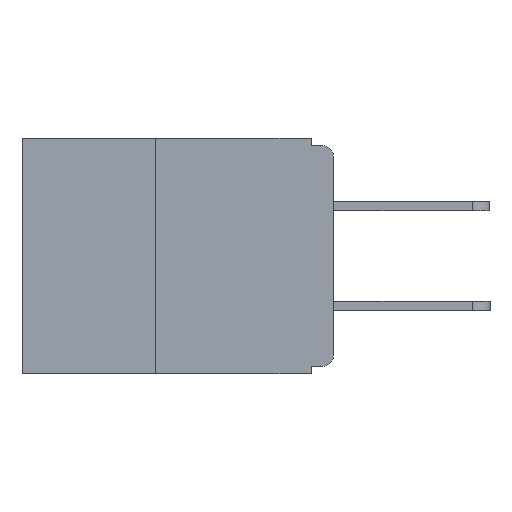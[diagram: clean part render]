
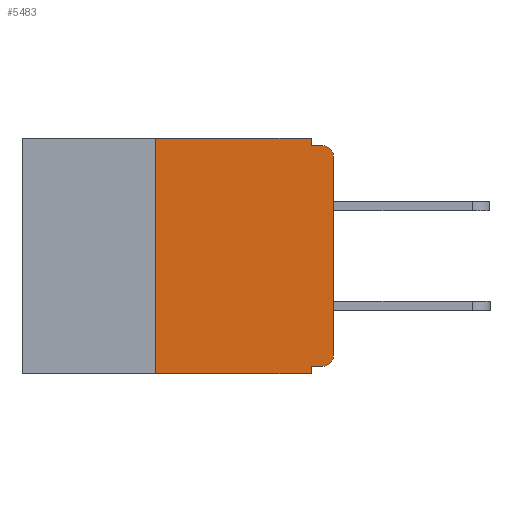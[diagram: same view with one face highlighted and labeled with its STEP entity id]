
A CAD part, left-side view. The second image highlights one B-rep face of the part: STEP entity #5483.
In plain terms, the highlighted planar face has unit normal (-1, 0, 0).
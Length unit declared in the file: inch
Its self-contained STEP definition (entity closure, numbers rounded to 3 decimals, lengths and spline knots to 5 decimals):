
#93 = EDGE_CURVE ( 'NONE', #1629, #9527, #11189, .T. ) ;
#175 = EDGE_CURVE ( 'NONE', #1629, #6311, #10903, .T. ) ;
#195 = AXIS2_PLACEMENT_3D ( 'NONE', #8005, #7891, #7655 ) ;
#348 = CARTESIAN_POINT ( 'NONE',  ( 0., 0.25, 0. ) ) ;
#1002 = CARTESIAN_POINT ( 'NONE',  ( 0., 0., -0.305 ) ) ;
#1053 = EDGE_CURVE ( 'NONE', #9122, #11343, #7869, .T. ) ;
#1329 = EDGE_CURVE ( 'NONE', #2762, #2732, #7465, .T. ) ;
#1629 = VERTEX_POINT ( 'NONE', #6068 ) ;
#1661 = AXIS2_PLACEMENT_3D ( 'NONE', #4460, #2580, #2341 ) ;
#1806 = VECTOR ( 'NONE', #8333, 39.37008 ) ;
#1836 = EDGE_CURVE ( 'NONE', #3424, #6311, #6360, .T. ) ;
#1947 = LINE ( 'NONE', #6629, #1806 ) ;
#2341 = DIRECTION ( 'NONE',  ( 0., 0., -1. ) ) ;
#2580 = DIRECTION ( 'NONE',  ( 1., 0., 0. ) ) ;
#2732 = VERTEX_POINT ( 'NONE', #11090 ) ;
#2762 = VERTEX_POINT ( 'NONE', #10242 ) ;
#2936 = DIRECTION ( 'NONE',  ( 0., 0., 1. ) ) ;
#3141 = ORIENTED_EDGE ( 'NONE', *, *, #1836, .F. ) ;
#3287 = VERTEX_POINT ( 'NONE', #11922 ) ;
#3313 = CARTESIAN_POINT ( 'NONE',  ( 0., 0.437, -0.33 ) ) ;
#3424 = VERTEX_POINT ( 'NONE', #4316 ) ;
#3521 = EDGE_CURVE ( 'NONE', #9527, #9820, #1947, .T. ) ;
#3797 = ORIENTED_EDGE ( 'NONE', *, *, #175, .T. ) ;
#4178 = EDGE_CURVE ( 'NONE', #9122, #3424, #12472, .T. ) ;
#4255 = EDGE_CURVE ( 'NONE', #11343, #3287, #12326, .T. ) ;
#4316 = CARTESIAN_POINT ( 'NONE',  ( 0., 0.031, -0.32 ) ) ;
#4460 = CARTESIAN_POINT ( 'NONE',  ( 0., 0.437, 0. ) ) ;
#4628 = PLANE ( 'NONE',  #1661 ) ;
#5052 = CARTESIAN_POINT ( 'NONE',  ( 0., 0.015, -0.32 ) ) ;
#5068 = ORIENTED_EDGE ( 'NONE', *, *, #93, .F. ) ;
#5282 = DIRECTION ( 'NONE',  ( 0., -1., 0. ) ) ;
#5483 = ADVANCED_FACE ( 'NONE', ( #10909 ), #4628, .F. ) ;
#5704 = ORIENTED_EDGE ( 'NONE', *, *, #3521, .F. ) ;
#6004 = CIRCLE ( 'NONE', #195, 0.015 ) ;
#6068 = CARTESIAN_POINT ( 'NONE',  ( 0., 0.25, -0.33 ) ) ;
#6297 = VECTOR ( 'NONE', #10953, 39.37008 ) ;
#6311 = VERTEX_POINT ( 'NONE', #8565 ) ;
#6360 = LINE ( 'NONE', #11053, #6297 ) ;
#6494 = CARTESIAN_POINT ( 'NONE',  ( 0., 0., 0. ) ) ;
#6629 = CARTESIAN_POINT ( 'NONE',  ( 0., 0.437, 0. ) ) ;
#7325 = DIRECTION ( 'NONE',  ( 0., 0., 1. ) ) ;
#7328 = VECTOR ( 'NONE', #11409, 39.37008 ) ;
#7465 = LINE ( 'NONE', #7972, #7328 ) ;
#7485 = CARTESIAN_POINT ( 'NONE',  ( 0., 0.031, 0. ) ) ;
#7655 = DIRECTION ( 'NONE',  ( 0., 0., -1. ) ) ;
#7687 = DIRECTION ( 'NONE',  ( 0., 0., -1. ) ) ;
#7869 = CIRCLE ( 'NONE', #8431, 0.015 ) ;
#7873 = ORIENTED_EDGE ( 'NONE', *, *, #11995, .F. ) ;
#7891 = DIRECTION ( 'NONE',  ( -1., 0., 0. ) ) ;
#7972 = CARTESIAN_POINT ( 'NONE',  ( 0., 0., -0.01 ) ) ;
#8005 = CARTESIAN_POINT ( 'NONE',  ( 0., 0.015, -0.025 ) ) ;
#8132 = DIRECTION ( 'NONE',  ( -1., 0., 0. ) ) ;
#8212 = ORIENTED_EDGE ( 'NONE', *, *, #8275, .T. ) ;
#8275 = EDGE_CURVE ( 'NONE', #3287, #2732, #6004, .T. ) ;
#8318 = CARTESIAN_POINT ( 'NONE',  ( 0., 0.031, 0. ) ) ;
#8333 = DIRECTION ( 'NONE',  ( 0., -1., 0. ) ) ;
#8334 = ORIENTED_EDGE ( 'NONE', *, *, #1053, .T. ) ;
#8431 = AXIS2_PLACEMENT_3D ( 'NONE', #8683, #8132, #8979 ) ;
#8565 = CARTESIAN_POINT ( 'NONE',  ( 0., 0.031, -0.33 ) ) ;
#8683 = CARTESIAN_POINT ( 'NONE',  ( 0., 0.015, -0.305 ) ) ;
#8973 = ORIENTED_EDGE ( 'NONE', *, *, #1329, .F. ) ;
#8979 = DIRECTION ( 'NONE',  ( 0., 0., -1. ) ) ;
#8985 = ORIENTED_EDGE ( 'NONE', *, *, #4255, .T. ) ;
#9122 = VERTEX_POINT ( 'NONE', #5052 ) ;
#9527 = VERTEX_POINT ( 'NONE', #348 ) ;
#9820 = VERTEX_POINT ( 'NONE', #7485 ) ;
#10242 = CARTESIAN_POINT ( 'NONE',  ( 0., 0.031, -0.01 ) ) ;
#10701 = EDGE_LOOP ( 'NONE', ( #8985, #8212, #8973, #7873, #5704, #5068, #3797, #3141, #11382, #8334 ) ) ;
#10763 = VECTOR ( 'NONE', #5282, 39.37008 ) ;
#10861 = VECTOR ( 'NONE', #7687, 39.37008 ) ;
#10903 = LINE ( 'NONE', #3313, #10763 ) ;
#10909 = FACE_OUTER_BOUND ( 'NONE', #10701, .T. ) ;
#10953 = DIRECTION ( 'NONE',  ( 0., 0., -1. ) ) ;
#11053 = CARTESIAN_POINT ( 'NONE',  ( 0., 0.031, -0.33 ) ) ;
#11090 = CARTESIAN_POINT ( 'NONE',  ( 0., 0.015, -0.01 ) ) ;
#11189 = LINE ( 'NONE', #11361, #11210 ) ;
#11210 = VECTOR ( 'NONE', #7325, 39.37008 ) ;
#11343 = VERTEX_POINT ( 'NONE', #1002 ) ;
#11361 = CARTESIAN_POINT ( 'NONE',  ( 0., 0.25, -0.33 ) ) ;
#11382 = ORIENTED_EDGE ( 'NONE', *, *, #4178, .F. ) ;
#11409 = DIRECTION ( 'NONE',  ( 0., -1., 0. ) ) ;
#11922 = CARTESIAN_POINT ( 'NONE',  ( 0., 0., -0.025 ) ) ;
#11964 = LINE ( 'NONE', #8318, #10861 ) ;
#11995 = EDGE_CURVE ( 'NONE', #9820, #2762, #11964, .T. ) ;
#12244 = CARTESIAN_POINT ( 'NONE',  ( 0., 0., -0.32 ) ) ;
#12320 = VECTOR ( 'NONE', #2936, 39.37008 ) ;
#12326 = LINE ( 'NONE', #6494, #12320 ) ;
#12361 = DIRECTION ( 'NONE',  ( 0., 1., 0. ) ) ;
#12387 = VECTOR ( 'NONE', #12361, 39.37008 ) ;
#12472 = LINE ( 'NONE', #12244, #12387 ) ;
